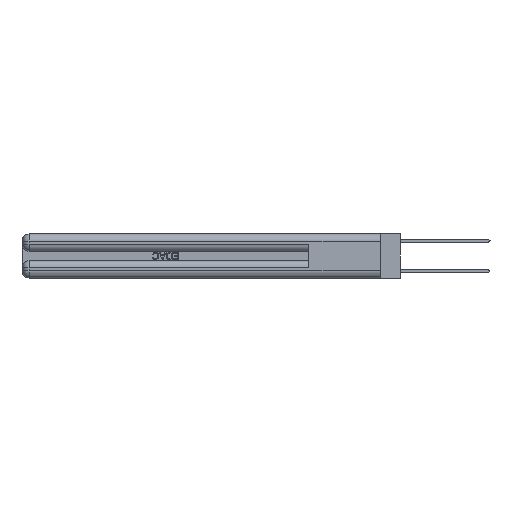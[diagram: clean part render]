
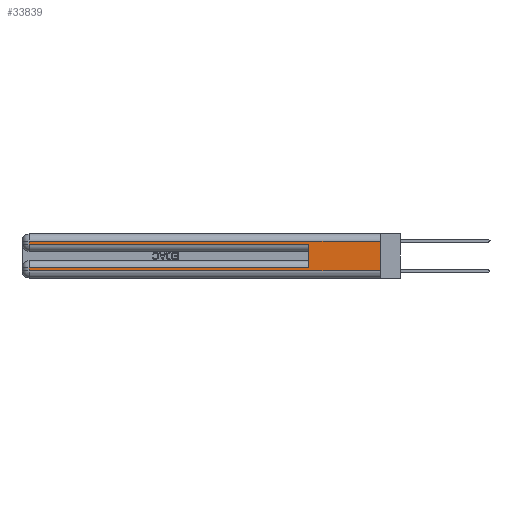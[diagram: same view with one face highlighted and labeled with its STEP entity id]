
A CAD part, left-side view. The second image highlights one B-rep face of the part: STEP entity #33839.
In plain terms, the highlighted planar face has unit normal (-1, 0, 0).
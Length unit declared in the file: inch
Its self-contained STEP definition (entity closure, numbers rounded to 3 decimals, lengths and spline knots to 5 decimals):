
#93 = CARTESIAN_POINT ( 'NONE',  ( 0., 2.94, 0.285 ) ) ;
#523 = LINE ( 'NONE', #15906, #36660 ) ;
#810 = DIRECTION ( 'NONE',  ( 0., 0., -1. ) ) ;
#2170 = VERTEX_POINT ( 'NONE', #14800 ) ;
#2819 = CARTESIAN_POINT ( 'NONE',  ( 0., 0.6, 0.285 ) ) ;
#3903 = ORIENTED_EDGE ( 'NONE', *, *, #22218, .F. ) ;
#4222 = DIRECTION ( 'NONE',  ( 0., 1., 0. ) ) ;
#5131 = CARTESIAN_POINT ( 'NONE',  ( 0., 0., 0.37 ) ) ;
#5696 = ORIENTED_EDGE ( 'NONE', *, *, #30252, .T. ) ;
#7521 = ORIENTED_EDGE ( 'NONE', *, *, #35970, .T. ) ;
#7790 = VERTEX_POINT ( 'NONE', #93 ) ;
#8003 = DIRECTION ( 'NONE',  ( 0., 0., -1. ) ) ;
#8479 = EDGE_CURVE ( 'NONE', #7790, #27480, #25434, .T. ) ;
#8546 = CARTESIAN_POINT ( 'NONE',  ( 0., 0., 0.37 ) ) ;
#9440 = VECTOR ( 'NONE', #11453, 39.37008 ) ;
#9850 = CARTESIAN_POINT ( 'NONE',  ( 0., 0., 0.085 ) ) ;
#10739 = VECTOR ( 'NONE', #810, 39.37008 ) ;
#11453 = DIRECTION ( 'NONE',  ( 0., 0., -1. ) ) ;
#12050 = ORIENTED_EDGE ( 'NONE', *, *, #33684, .T. ) ;
#12903 = DIRECTION ( 'NONE',  ( 0., 0., 1. ) ) ;
#13174 = DIRECTION ( 'NONE',  ( 0., -1., 0. ) ) ;
#13870 = VECTOR ( 'NONE', #4222, 39.37008 ) ;
#14070 = CARTESIAN_POINT ( 'NONE',  ( 0., 2.94, 0.06 ) ) ;
#14205 = VECTOR ( 'NONE', #12903, 39.37008 ) ;
#14461 = VERTEX_POINT ( 'NONE', #33964 ) ;
#14800 = CARTESIAN_POINT ( 'NONE',  ( 0., 0., 0.31 ) ) ;
#15586 = ORIENTED_EDGE ( 'NONE', *, *, #26590, .F. ) ;
#15643 = LINE ( 'NONE', #9850, #13870 ) ;
#15906 = CARTESIAN_POINT ( 'NONE',  ( 0., 0., 0.06 ) ) ;
#15953 = VERTEX_POINT ( 'NONE', #27035 ) ;
#16137 = VECTOR ( 'NONE', #35218, 39.37008 ) ;
#17229 = DIRECTION ( 'NONE',  ( 0., -1., 0. ) ) ;
#17808 = ORIENTED_EDGE ( 'NONE', *, *, #35845, .T. ) ;
#17906 = VECTOR ( 'NONE', #17229, 39.37008 ) ;
#18017 = AXIS2_PLACEMENT_3D ( 'NONE', #5131, #25085, #8003 ) ;
#19226 = LINE ( 'NONE', #20715, #10739 ) ;
#19600 = EDGE_CURVE ( 'NONE', #31506, #22174, #21626, .T. ) ;
#20715 = CARTESIAN_POINT ( 'NONE',  ( 0., 2.94, 0.37 ) ) ;
#21626 = LINE ( 'NONE', #30504, #35838 ) ;
#22174 = VERTEX_POINT ( 'NONE', #14070 ) ;
#22218 = EDGE_CURVE ( 'NONE', #2170, #30774, #32165, .T. ) ;
#25085 = DIRECTION ( 'NONE',  ( 1., 0., 0. ) ) ;
#25434 = LINE ( 'NONE', #25641, #17906 ) ;
#25641 = CARTESIAN_POINT ( 'NONE',  ( 0., 0., 0.285 ) ) ;
#26590 = EDGE_CURVE ( 'NONE', #15953, #27480, #36858, .T. ) ;
#27035 = CARTESIAN_POINT ( 'NONE',  ( 0., 0.6, 0.085 ) ) ;
#27480 = VERTEX_POINT ( 'NONE', #2819 ) ;
#27627 = DIRECTION ( 'NONE',  ( 0., 0., -1. ) ) ;
#29197 = CARTESIAN_POINT ( 'NONE',  ( 0., 2.94, 0.085 ) ) ;
#30252 = EDGE_CURVE ( 'NONE', #2170, #14461, #32131, .T. ) ;
#30504 = CARTESIAN_POINT ( 'NONE',  ( 0., 2.94, 0.37 ) ) ;
#30774 = VERTEX_POINT ( 'NONE', #34949 ) ;
#31335 = FACE_OUTER_BOUND ( 'NONE', #33191, .T. ) ;
#31506 = VERTEX_POINT ( 'NONE', #29197 ) ;
#32052 = ORIENTED_EDGE ( 'NONE', *, *, #19600, .T. ) ;
#32131 = LINE ( 'NONE', #32362, #16137 ) ;
#32165 = LINE ( 'NONE', #8546, #9440 ) ;
#32362 = CARTESIAN_POINT ( 'NONE',  ( 0., 0., 0.31 ) ) ;
#33191 = EDGE_LOOP ( 'NONE', ( #3903, #5696, #17808, #33806, #15586, #7521, #32052, #12050 ) ) ;
#33684 = EDGE_CURVE ( 'NONE', #22174, #30774, #523, .T. ) ;
#33806 = ORIENTED_EDGE ( 'NONE', *, *, #8479, .T. ) ;
#33839 = ADVANCED_FACE ( 'NONE', ( #31335 ), #36391, .F. ) ;
#33964 = CARTESIAN_POINT ( 'NONE',  ( 0., 2.94, 0.31 ) ) ;
#34949 = CARTESIAN_POINT ( 'NONE',  ( 0., 0., 0.06 ) ) ;
#35218 = DIRECTION ( 'NONE',  ( 0., 1., 0. ) ) ;
#35521 = CARTESIAN_POINT ( 'NONE',  ( 0., 0.6, 0.145 ) ) ;
#35838 = VECTOR ( 'NONE', #27627, 39.37008 ) ;
#35845 = EDGE_CURVE ( 'NONE', #14461, #7790, #19226, .T. ) ;
#35970 = EDGE_CURVE ( 'NONE', #15953, #31506, #15643, .T. ) ;
#36391 = PLANE ( 'NONE',  #18017 ) ;
#36660 = VECTOR ( 'NONE', #13174, 39.37008 ) ;
#36858 = LINE ( 'NONE', #35521, #14205 ) ;
